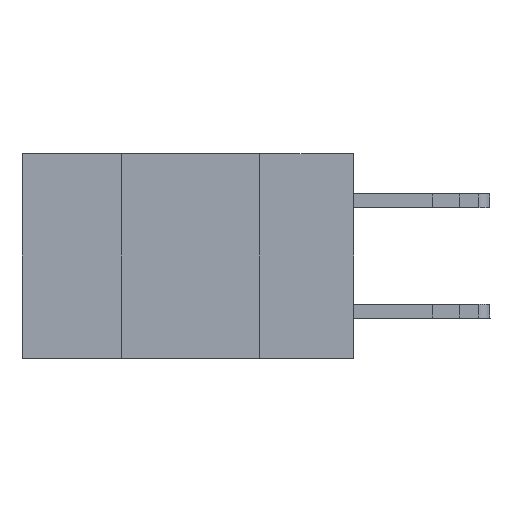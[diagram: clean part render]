
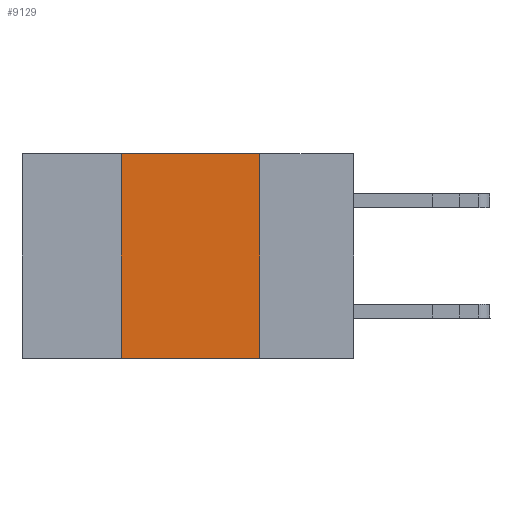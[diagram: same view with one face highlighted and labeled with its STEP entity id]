
A CAD part, left-side view. The second image highlights one B-rep face of the part: STEP entity #9129.
In plain terms, the highlighted planar face has unit normal (-1, 0, 0).
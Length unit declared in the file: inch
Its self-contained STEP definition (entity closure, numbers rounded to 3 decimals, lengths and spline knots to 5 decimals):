
#363 = AXIS2_PLACEMENT_3D ( 'NONE', #13198, #9923, #21570 ) ;
#2844 = LINE ( 'NONE', #8350, #18344 ) ;
#3613 = CARTESIAN_POINT ( 'NONE',  ( 0., 0.17, 0. ) ) ;
#3893 = ORIENTED_EDGE ( 'NONE', *, *, #19546, .F. ) ;
#4015 = ORIENTED_EDGE ( 'NONE', *, *, #16821, .F. ) ;
#4727 = ORIENTED_EDGE ( 'NONE', *, *, #21696, .F. ) ;
#4859 = ORIENTED_EDGE ( 'NONE', *, *, #18648, .T. ) ;
#5954 = VECTOR ( 'NONE', #20362, 39.37008 ) ;
#7018 = LINE ( 'NONE', #18678, #5954 ) ;
#7643 = DIRECTION ( 'NONE',  ( 0., -1., 0. ) ) ;
#7850 = LINE ( 'NONE', #17553, #16621 ) ;
#8350 = CARTESIAN_POINT ( 'NONE',  ( 0., 0.42, 0. ) ) ;
#9129 = ADVANCED_FACE ( 'NONE', ( #14035 ), #14874, .F. ) ;
#9923 = DIRECTION ( 'NONE',  ( 1., 0., 0. ) ) ;
#10390 = CARTESIAN_POINT ( 'NONE',  ( 0., 0.42, 0. ) ) ;
#10906 = CARTESIAN_POINT ( 'NONE',  ( 0., 0.17, -0.37 ) ) ;
#12020 = VERTEX_POINT ( 'NONE', #16203 ) ;
#12742 = DIRECTION ( 'NONE',  ( 0., -1., 0. ) ) ;
#13198 = CARTESIAN_POINT ( 'NONE',  ( 0., 0.6, 0. ) ) ;
#13635 = VERTEX_POINT ( 'NONE', #3613 ) ;
#14035 = FACE_OUTER_BOUND ( 'NONE', #21467, .T. ) ;
#14874 = PLANE ( 'NONE',  #363 ) ;
#15450 = LINE ( 'NONE', #21058, #19358 ) ;
#16203 = CARTESIAN_POINT ( 'NONE',  ( 0., 0.42, -0.37 ) ) ;
#16621 = VECTOR ( 'NONE', #7643, 39.37008 ) ;
#16821 = EDGE_CURVE ( 'NONE', #21858, #13635, #15450, .T. ) ;
#17553 = CARTESIAN_POINT ( 'NONE',  ( 0., 0.6, -0.37 ) ) ;
#18344 = VECTOR ( 'NONE', #21621, 39.37008 ) ;
#18648 = EDGE_CURVE ( 'NONE', #12020, #21498, #7850, .T. ) ;
#18678 = CARTESIAN_POINT ( 'NONE',  ( 0., 0.17, 0. ) ) ;
#19358 = VECTOR ( 'NONE', #12742, 39.37008 ) ;
#19546 = EDGE_CURVE ( 'NONE', #13635, #21498, #7018, .T. ) ;
#20362 = DIRECTION ( 'NONE',  ( 0., 0., -1. ) ) ;
#21058 = CARTESIAN_POINT ( 'NONE',  ( 0., 0.6, 0. ) ) ;
#21467 = EDGE_LOOP ( 'NONE', ( #3893, #4015, #4727, #4859 ) ) ;
#21498 = VERTEX_POINT ( 'NONE', #10906 ) ;
#21570 = DIRECTION ( 'NONE',  ( 0., 0., -1. ) ) ;
#21621 = DIRECTION ( 'NONE',  ( 0., 0., 1. ) ) ;
#21696 = EDGE_CURVE ( 'NONE', #12020, #21858, #2844, .T. ) ;
#21858 = VERTEX_POINT ( 'NONE', #10390 ) ;
